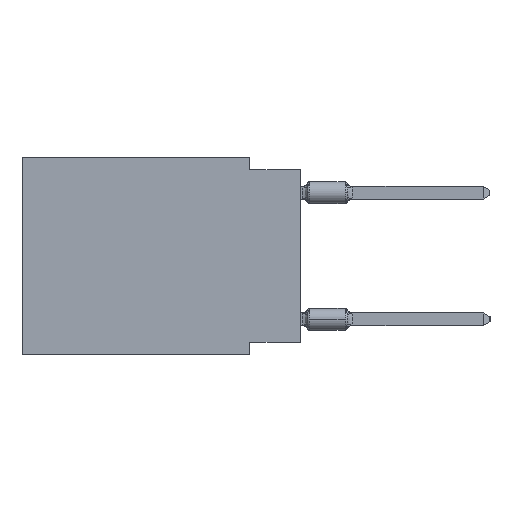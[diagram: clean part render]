
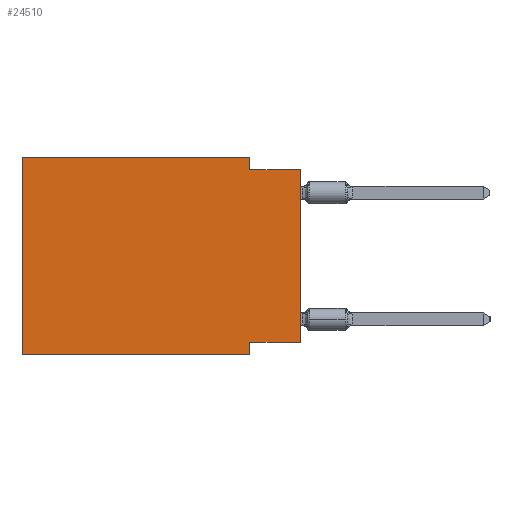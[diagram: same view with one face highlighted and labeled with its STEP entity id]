
A CAD part, left-side view. The second image highlights one B-rep face of the part: STEP entity #24510.
In plain terms, the highlighted planar face has unit normal (-1, 0, 0).
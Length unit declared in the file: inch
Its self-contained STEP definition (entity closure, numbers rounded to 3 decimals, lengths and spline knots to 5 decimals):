
#527 = VECTOR ( 'NONE', #20548, 39.37008 ) ;
#839 = LINE ( 'NONE', #23879, #41328 ) ;
#1978 = DIRECTION ( 'NONE',  ( 0., -1., 0. ) ) ;
#2836 = CARTESIAN_POINT ( 'NONE',  ( 0., 0.55, 0. ) ) ;
#2973 = LINE ( 'NONE', #43100, #38191 ) ;
#2984 = ORIENTED_EDGE ( 'NONE', *, *, #8859, .T. ) ;
#3318 = VERTEX_POINT ( 'NONE', #17462 ) ;
#3555 = VECTOR ( 'NONE', #30116, 39.37008 ) ;
#4848 = CARTESIAN_POINT ( 'NONE',  ( 0., 0.55, -0.39 ) ) ;
#4906 = LINE ( 'NONE', #18426, #22972 ) ;
#5426 = PLANE ( 'NONE',  #38885 ) ;
#5858 = VERTEX_POINT ( 'NONE', #35946 ) ;
#5911 = LINE ( 'NONE', #2836, #22724 ) ;
#6440 = ORIENTED_EDGE ( 'NONE', *, *, #39183, .F. ) ;
#7247 = LINE ( 'NONE', #17230, #33761 ) ;
#7972 = LINE ( 'NONE', #21276, #10538 ) ;
#8733 = ORIENTED_EDGE ( 'NONE', *, *, #23811, .F. ) ;
#8859 = EDGE_CURVE ( 'NONE', #28528, #26679, #26796, .T. ) ;
#9524 = CARTESIAN_POINT ( 'NONE',  ( 0., 0.55, -0.39 ) ) ;
#9775 = ORIENTED_EDGE ( 'NONE', *, *, #42536, .F. ) ;
#10369 = DIRECTION ( 'NONE',  ( 0., 0., -1. ) ) ;
#10538 = VECTOR ( 'NONE', #21924, 39.37008 ) ;
#11881 = EDGE_LOOP ( 'NONE', ( #22899, #6440, #25637, #35619, #32630, #2984, #9775, #8733 ) ) ;
#13347 = CARTESIAN_POINT ( 'NONE',  ( 0., 0.1, 0. ) ) ;
#13744 = EDGE_CURVE ( 'NONE', #3318, #5858, #4906, .T. ) ;
#14451 = EDGE_CURVE ( 'NONE', #18191, #41476, #839, .T. ) ;
#15400 = CARTESIAN_POINT ( 'NONE',  ( 0., 0.55, 0. ) ) ;
#15516 = CARTESIAN_POINT ( 'NONE',  ( 0., 0.1, -0.39 ) ) ;
#17230 = CARTESIAN_POINT ( 'NONE',  ( 0., 0.55, 0. ) ) ;
#17268 = VERTEX_POINT ( 'NONE', #19428 ) ;
#17462 = CARTESIAN_POINT ( 'NONE',  ( 0., 0., -0.365 ) ) ;
#18191 = VERTEX_POINT ( 'NONE', #13347 ) ;
#18426 = CARTESIAN_POINT ( 'NONE',  ( 0., 0., 0. ) ) ;
#18718 = DIRECTION ( 'NONE',  ( 0., 0., -1. ) ) ;
#19275 = DIRECTION ( 'NONE',  ( 0., 0., 1. ) ) ;
#19428 = CARTESIAN_POINT ( 'NONE',  ( 0., 0.55, 0. ) ) ;
#20548 = DIRECTION ( 'NONE',  ( 0., -1., 0. ) ) ;
#20894 = CARTESIAN_POINT ( 'NONE',  ( 0., 0.1, -0.025 ) ) ;
#21276 = CARTESIAN_POINT ( 'NONE',  ( 0., 0., -0.365 ) ) ;
#21400 = DIRECTION ( 'NONE',  ( 1., 0., 0. ) ) ;
#21924 = DIRECTION ( 'NONE',  ( 0., 1., 0. ) ) ;
#22724 = VECTOR ( 'NONE', #1978, 39.37008 ) ;
#22899 = ORIENTED_EDGE ( 'NONE', *, *, #13744, .T. ) ;
#22972 = VECTOR ( 'NONE', #19275, 39.37008 ) ;
#23811 = EDGE_CURVE ( 'NONE', #3318, #31120, #7972, .T. ) ;
#23879 = CARTESIAN_POINT ( 'NONE',  ( 0., 0.1, 0. ) ) ;
#24319 = LINE ( 'NONE', #37836, #527 ) ;
#24510 = ADVANCED_FACE ( 'NONE', ( #34906 ), #5426, .F. ) ;
#25637 = ORIENTED_EDGE ( 'NONE', *, *, #14451, .F. ) ;
#26241 = DIRECTION ( 'NONE',  ( 0., 0., -1. ) ) ;
#26679 = VERTEX_POINT ( 'NONE', #15516 ) ;
#26796 = LINE ( 'NONE', #9524, #3555 ) ;
#27173 = EDGE_CURVE ( 'NONE', #17268, #18191, #5911, .T. ) ;
#28528 = VERTEX_POINT ( 'NONE', #4848 ) ;
#30116 = DIRECTION ( 'NONE',  ( 0., -1., 0. ) ) ;
#31093 = CARTESIAN_POINT ( 'NONE',  ( 0., 0.1, -0.365 ) ) ;
#31120 = VERTEX_POINT ( 'NONE', #31093 ) ;
#32630 = ORIENTED_EDGE ( 'NONE', *, *, #39110, .F. ) ;
#33761 = VECTOR ( 'NONE', #37175, 39.37008 ) ;
#34906 = FACE_OUTER_BOUND ( 'NONE', #11881, .T. ) ;
#35619 = ORIENTED_EDGE ( 'NONE', *, *, #27173, .F. ) ;
#35946 = CARTESIAN_POINT ( 'NONE',  ( 0., 0., -0.025 ) ) ;
#37175 = DIRECTION ( 'NONE',  ( 0., 0., 1. ) ) ;
#37836 = CARTESIAN_POINT ( 'NONE',  ( 0., 0., -0.025 ) ) ;
#38191 = VECTOR ( 'NONE', #26241, 39.37008 ) ;
#38885 = AXIS2_PLACEMENT_3D ( 'NONE', #15400, #21400, #18718 ) ;
#39110 = EDGE_CURVE ( 'NONE', #28528, #17268, #7247, .T. ) ;
#39183 = EDGE_CURVE ( 'NONE', #41476, #5858, #24319, .T. ) ;
#41328 = VECTOR ( 'NONE', #10369, 39.37008 ) ;
#41476 = VERTEX_POINT ( 'NONE', #20894 ) ;
#42536 = EDGE_CURVE ( 'NONE', #31120, #26679, #2973, .T. ) ;
#43100 = CARTESIAN_POINT ( 'NONE',  ( 0., 0.1, -0.39 ) ) ;
